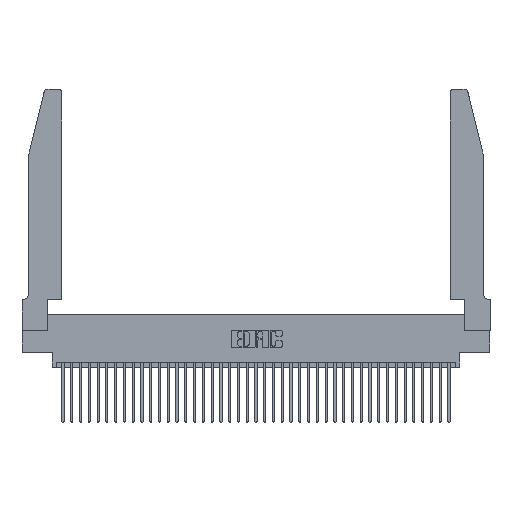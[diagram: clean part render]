
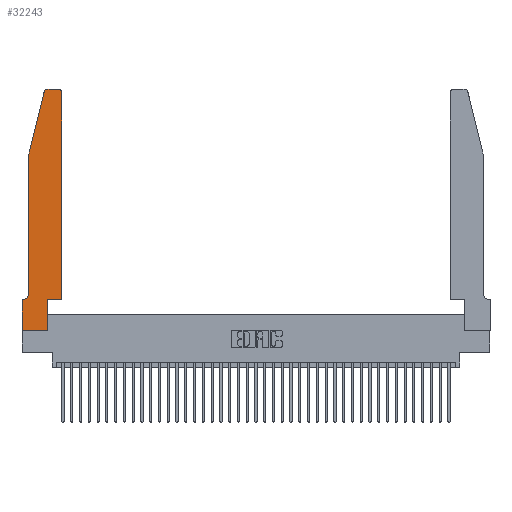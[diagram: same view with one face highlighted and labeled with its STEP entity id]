
A CAD part, top view. The second image highlights one B-rep face of the part: STEP entity #32243.
In plain terms, the highlighted planar face has unit normal (0, 0, 1).
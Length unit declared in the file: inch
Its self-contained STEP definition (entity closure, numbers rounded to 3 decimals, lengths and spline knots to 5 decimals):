
#323 = CARTESIAN_POINT ( 'NONE',  ( 0.4505, 0.35, 0.37 ) ) ;
#447 = CARTESIAN_POINT ( 'NONE',  ( 0.25487, 2.72718, 0.37 ) ) ;
#1404 = CARTESIAN_POINT ( 'NONE',  ( 0.0055, 0.42, 0.37 ) ) ;
#1452 = CARTESIAN_POINT ( 'NONE',  ( 0.284, 2.75, 0.37 ) ) ;
#1641 = VERTEX_POINT ( 'NONE', #36208 ) ;
#1755 = CARTESIAN_POINT ( 'NONE',  ( 0.4205, 2.72, 0.37 ) ) ;
#1896 = CARTESIAN_POINT ( 'NONE',  ( 0.4505, 0.35, 0.37 ) ) ;
#2036 = VERTEX_POINT ( 'NONE', #17883 ) ;
#2149 = LINE ( 'NONE', #9680, #38725 ) ;
#2534 = ORIENTED_EDGE ( 'NONE', *, *, #39196, .T. ) ;
#2734 = VERTEX_POINT ( 'NONE', #6543 ) ;
#3397 = VECTOR ( 'NONE', #17961, 39.37008 ) ;
#3866 = DIRECTION ( 'NONE',  ( 0., 1., 0. ) ) ;
#3897 = CIRCLE ( 'NONE', #11205, 0.03 ) ;
#4062 = LINE ( 'NONE', #22103, #11731 ) ;
#4137 = CARTESIAN_POINT ( 'NONE',  ( 0.2865, 0.35, 0.37 ) ) ;
#4434 = CIRCLE ( 'NONE', #34257, 0.07 ) ;
#5098 = DIRECTION ( 'NONE',  ( 1., 0., 0. ) ) ;
#5378 = CARTESIAN_POINT ( 'NONE',  ( 0.4505, 2.72, 0.37 ) ) ;
#5666 = DIRECTION ( 'NONE',  ( 1., 0., 0. ) ) ;
#6284 = DIRECTION ( 'NONE',  ( 0., 1., 0. ) ) ;
#6481 = EDGE_CURVE ( 'NONE', #38599, #24818, #4434, .T. ) ;
#6543 = CARTESIAN_POINT ( 'NONE',  ( 0.2865, 0.35, 0.37 ) ) ;
#7980 = ORIENTED_EDGE ( 'NONE', *, *, #28599, .T. ) ;
#8081 = VECTOR ( 'NONE', #17168, 39.37008 ) ;
#8571 = VERTEX_POINT ( 'NONE', #447 ) ;
#8897 = ORIENTED_EDGE ( 'NONE', *, *, #21756, .T. ) ;
#9680 = CARTESIAN_POINT ( 'NONE',  ( 0.0755, 2., 0.37 ) ) ;
#9865 = LINE ( 'NONE', #38434, #18026 ) ;
#9919 = CARTESIAN_POINT ( 'NONE',  ( 0., 0.35, 0.37 ) ) ;
#10082 = LINE ( 'NONE', #323, #16286 ) ;
#10556 = VERTEX_POINT ( 'NONE', #17501 ) ;
#11205 = AXIS2_PLACEMENT_3D ( 'NONE', #1755, #17428, #5098 ) ;
#11731 = VECTOR ( 'NONE', #28429, 39.37008 ) ;
#12088 = ORIENTED_EDGE ( 'NONE', *, *, #32888, .T. ) ;
#12335 = VERTEX_POINT ( 'NONE', #24932 ) ;
#14801 = CIRCLE ( 'NONE', #22877, 0.03 ) ;
#16016 = EDGE_CURVE ( 'NONE', #12335, #38599, #2149, .T. ) ;
#16286 = VECTOR ( 'NONE', #6284, 39.37008 ) ;
#17168 = DIRECTION ( 'NONE',  ( 1., 0., 0. ) ) ;
#17265 = EDGE_CURVE ( 'NONE', #19277, #8571, #14801, .T. ) ;
#17270 = CARTESIAN_POINT ( 'NONE',  ( 0., 0.35, 0.37 ) ) ;
#17428 = DIRECTION ( 'NONE',  ( 0., 0., 1. ) ) ;
#17501 = CARTESIAN_POINT ( 'NONE',  ( 0.2865, 0., 0.37 ) ) ;
#17608 = VERTEX_POINT ( 'NONE', #5378 ) ;
#17731 = ORIENTED_EDGE ( 'NONE', *, *, #23107, .T. ) ;
#17883 = CARTESIAN_POINT ( 'NONE',  ( 0., 0., 0.37 ) ) ;
#17961 = DIRECTION ( 'NONE',  ( -1., 0., 0. ) ) ;
#18026 = VECTOR ( 'NONE', #28855, 39.37008 ) ;
#18520 = LINE ( 'NONE', #4137, #32515 ) ;
#18823 = ORIENTED_EDGE ( 'NONE', *, *, #30668, .T. ) ;
#19024 = ORIENTED_EDGE ( 'NONE', *, *, #6481, .T. ) ;
#19277 = VERTEX_POINT ( 'NONE', #1452 ) ;
#20196 = ORIENTED_EDGE ( 'NONE', *, *, #16016, .T. ) ;
#20760 = VECTOR ( 'NONE', #5666, 39.37008 ) ;
#20938 = AXIS2_PLACEMENT_3D ( 'NONE', #17270, #23861, #29802 ) ;
#21078 = LINE ( 'NONE', #1896, #8081 ) ;
#21332 = ORIENTED_EDGE ( 'NONE', *, *, #17265, .T. ) ;
#21715 = VERTEX_POINT ( 'NONE', #39175 ) ;
#21756 = EDGE_CURVE ( 'NONE', #2036, #10556, #22189, .T. ) ;
#22103 = CARTESIAN_POINT ( 'NONE',  ( 0., 0., 0.37 ) ) ;
#22189 = LINE ( 'NONE', #24079, #20760 ) ;
#22195 = VECTOR ( 'NONE', #35667, 39.37008 ) ;
#22271 = FACE_OUTER_BOUND ( 'NONE', #39137, .T. ) ;
#22576 = DIRECTION ( 'NONE',  ( 0., -1., 0. ) ) ;
#22877 = AXIS2_PLACEMENT_3D ( 'NONE', #25532, #28640, #34437 ) ;
#22977 = CARTESIAN_POINT ( 'NONE',  ( 0.0755, 0.42, 0.37 ) ) ;
#23107 = EDGE_CURVE ( 'NONE', #1641, #17608, #10082, .T. ) ;
#23861 = DIRECTION ( 'NONE',  ( 0., 0., 1. ) ) ;
#24079 = CARTESIAN_POINT ( 'NONE',  ( 0., 0., 0.37 ) ) ;
#24158 = CARTESIAN_POINT ( 'NONE',  ( 0.2605, 2.75, 0.37 ) ) ;
#24538 = ORIENTED_EDGE ( 'NONE', *, *, #26917, .T. ) ;
#24818 = VERTEX_POINT ( 'NONE', #36160 ) ;
#24905 = ORIENTED_EDGE ( 'NONE', *, *, #30012, .T. ) ;
#24932 = CARTESIAN_POINT ( 'NONE',  ( 0.0755, 2., 0.37 ) ) ;
#25532 = CARTESIAN_POINT ( 'NONE',  ( 0.284, 2.72, 0.37 ) ) ;
#26373 = CARTESIAN_POINT ( 'NONE',  ( 0.0755, 2., 0.37 ) ) ;
#26745 = EDGE_CURVE ( 'NONE', #17608, #21715, #3897, .T. ) ;
#26917 = EDGE_CURVE ( 'NONE', #21715, #19277, #29410, .T. ) ;
#28429 = DIRECTION ( 'NONE',  ( 0., -1., 0. ) ) ;
#28599 = EDGE_CURVE ( 'NONE', #2734, #1641, #21078, .T. ) ;
#28640 = DIRECTION ( 'NONE',  ( 0., 0., 1. ) ) ;
#28855 = DIRECTION ( 'NONE',  ( -1., 0., 0. ) ) ;
#29211 = DIRECTION ( 'NONE',  ( 0., 0., -1. ) ) ;
#29343 = DIRECTION ( 'NONE',  ( -1., 0., 0. ) ) ;
#29410 = LINE ( 'NONE', #24158, #3397 ) ;
#29665 = PLANE ( 'NONE',  #20938 ) ;
#29802 = DIRECTION ( 'NONE',  ( 1., 0., 0. ) ) ;
#30012 = EDGE_CURVE ( 'NONE', #10556, #2734, #18520, .T. ) ;
#30668 = EDGE_CURVE ( 'NONE', #31984, #2036, #4062, .T. ) ;
#31895 = ORIENTED_EDGE ( 'NONE', *, *, #26745, .T. ) ;
#31984 = VERTEX_POINT ( 'NONE', #9919 ) ;
#32243 = ADVANCED_FACE ( 'NONE', ( #22271 ), #29665, .T. ) ;
#32515 = VECTOR ( 'NONE', #3866, 39.37008 ) ;
#32888 = EDGE_CURVE ( 'NONE', #8571, #12335, #38618, .T. ) ;
#34257 = AXIS2_PLACEMENT_3D ( 'NONE', #1404, #29211, #29343 ) ;
#34437 = DIRECTION ( 'NONE',  ( 1., 0., 0. ) ) ;
#35667 = DIRECTION ( 'NONE',  ( -0.239, -0.971, 0. ) ) ;
#36160 = CARTESIAN_POINT ( 'NONE',  ( 0.0055, 0.35, 0.37 ) ) ;
#36208 = CARTESIAN_POINT ( 'NONE',  ( 0.4505, 0.35, 0.37 ) ) ;
#38434 = CARTESIAN_POINT ( 'NONE',  ( 0.0755, 0.35, 0.37 ) ) ;
#38599 = VERTEX_POINT ( 'NONE', #22977 ) ;
#38618 = LINE ( 'NONE', #26373, #22195 ) ;
#38725 = VECTOR ( 'NONE', #22576, 39.37008 ) ;
#39137 = EDGE_LOOP ( 'NONE', ( #24538, #21332, #12088, #20196, #19024, #2534, #18823, #8897, #24905, #7980, #17731, #31895 ) ) ;
#39175 = CARTESIAN_POINT ( 'NONE',  ( 0.4205, 2.75, 0.37 ) ) ;
#39196 = EDGE_CURVE ( 'NONE', #24818, #31984, #9865, .T. ) ;
